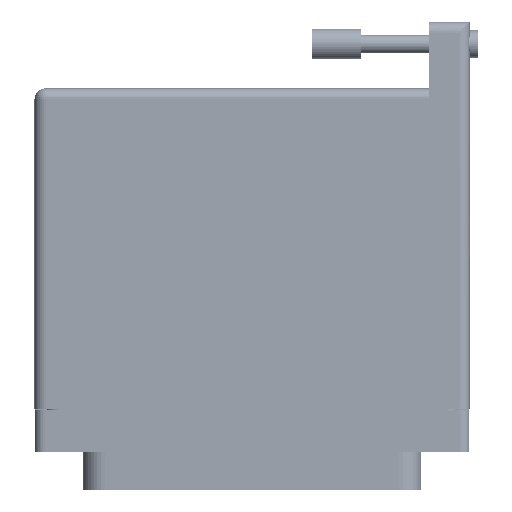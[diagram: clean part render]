
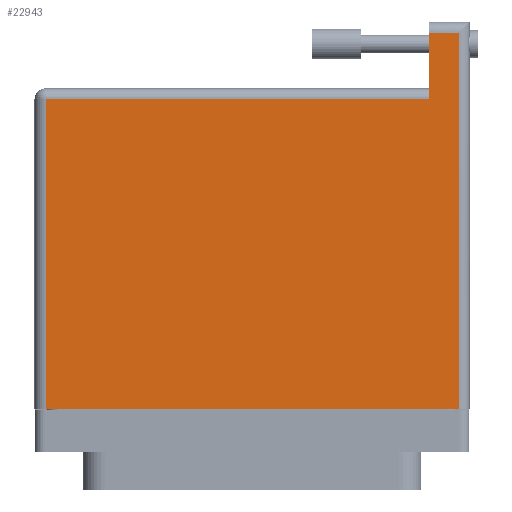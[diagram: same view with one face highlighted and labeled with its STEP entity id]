
A CAD part, front view. The second image highlights one B-rep face of the part: STEP entity #22943.
In plain terms, the highlighted face is planar.
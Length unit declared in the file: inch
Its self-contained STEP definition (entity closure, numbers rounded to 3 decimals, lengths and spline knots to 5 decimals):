
#1358 = DIRECTION ( 'NONE',  ( -1., 0., 0. ) ) ;
#3058 = DIRECTION ( 'NONE',  ( 1., 0., 0. ) ) ;
#5141 = LINE ( 'NONE', #35611, #28770 ) ;
#5504 = CARTESIAN_POINT ( 'NONE',  ( 1.1215, 2.35, 0.765 ) ) ;
#7513 = ORIENTED_EDGE ( 'NONE', *, *, #45523, .T. ) ;
#9622 = VERTEX_POINT ( 'NONE', #56872 ) ;
#10541 = VECTOR ( 'NONE', #24838, 39.37008 ) ;
#12501 = EDGE_LOOP ( 'NONE', ( #52938, #48345, #7513, #20929, #66838, #85293 ) ) ;
#14203 = EDGE_CURVE ( 'NONE', #26260, #32642, #77189, .T. ) ;
#15329 = VERTEX_POINT ( 'NONE', #57240 ) ;
#15358 = VERTEX_POINT ( 'NONE', #23186 ) ;
#20002 = CARTESIAN_POINT ( 'NONE',  ( -1.3075, -0.1, 0.765 ) ) ;
#20929 = ORIENTED_EDGE ( 'NONE', *, *, #73309, .T. ) ;
#22371 = LINE ( 'NONE', #20002, #75187 ) ;
#22452 = CARTESIAN_POINT ( 'NONE',  ( -1.3075, 1.86, 0.765 ) ) ;
#22943 = ADVANCED_FACE ( 'NONE', ( #50663 ), #32079, .F. ) ;
#23186 = CARTESIAN_POINT ( 'NONE',  ( -1.3075, -0.1, 0.765 ) ) ;
#24838 = DIRECTION ( 'NONE',  ( 0., 1., 0. ) ) ;
#25128 = CARTESIAN_POINT ( 'NONE',  ( 1.3075, 2.35, 0.765 ) ) ;
#25647 = CARTESIAN_POINT ( 'NONE',  ( 1.1215, 2.28, 0.765 ) ) ;
#26260 = VERTEX_POINT ( 'NONE', #25647 ) ;
#26635 = DIRECTION ( 'NONE',  ( 0., -1., 0. ) ) ;
#27001 = EDGE_CURVE ( 'NONE', #9622, #26260, #54856, .T. ) ;
#28770 = VECTOR ( 'NONE', #1358, 39.37008 ) ;
#30383 = CARTESIAN_POINT ( 'NONE',  ( -1.3775, -0.1, 0.765 ) ) ;
#32079 = PLANE ( 'NONE',  #88603 ) ;
#32642 = VERTEX_POINT ( 'NONE', #76925 ) ;
#35611 = CARTESIAN_POINT ( 'NONE',  ( -1.3775, 1.86, 0.765 ) ) ;
#39358 = DIRECTION ( 'NONE',  ( -1., 0., 0. ) ) ;
#45307 = EDGE_CURVE ( 'NONE', #15329, #9622, #74166, .T. ) ;
#45523 = EDGE_CURVE ( 'NONE', #67258, #15358, #22371, .T. ) ;
#45669 = EDGE_CURVE ( 'NONE', #32642, #67258, #5141, .T. ) ;
#47859 = DIRECTION ( 'NONE',  ( -1., 0., 0. ) ) ;
#48345 = ORIENTED_EDGE ( 'NONE', *, *, #45669, .T. ) ;
#50663 = FACE_OUTER_BOUND ( 'NONE', #12501, .T. ) ;
#52444 = VECTOR ( 'NONE', #53622, 39.37008 ) ;
#52692 = VECTOR ( 'NONE', #47859, 39.37008 ) ;
#52866 = CARTESIAN_POINT ( 'NONE',  ( -1.3775, 1.93, 0.765 ) ) ;
#52938 = ORIENTED_EDGE ( 'NONE', *, *, #14203, .T. ) ;
#53622 = DIRECTION ( 'NONE',  ( 0., -1., 0. ) ) ;
#54856 = LINE ( 'NONE', #62279, #52692 ) ;
#56872 = CARTESIAN_POINT ( 'NONE',  ( 1.3075, 2.28, 0.765 ) ) ;
#57240 = CARTESIAN_POINT ( 'NONE',  ( 1.3075, -0.1, 0.765 ) ) ;
#62279 = CARTESIAN_POINT ( 'NONE',  ( -1.3775, 2.28, 0.765 ) ) ;
#64922 = LINE ( 'NONE', #30383, #72473 ) ;
#66738 = DIRECTION ( 'NONE',  ( 0., 0., -1. ) ) ;
#66838 = ORIENTED_EDGE ( 'NONE', *, *, #45307, .T. ) ;
#67258 = VERTEX_POINT ( 'NONE', #22452 ) ;
#72473 = VECTOR ( 'NONE', #3058, 39.37008 ) ;
#73309 = EDGE_CURVE ( 'NONE', #15358, #15329, #64922, .T. ) ;
#74166 = LINE ( 'NONE', #25128, #10541 ) ;
#75187 = VECTOR ( 'NONE', #26635, 39.37008 ) ;
#76925 = CARTESIAN_POINT ( 'NONE',  ( 1.1215, 1.86, 0.765 ) ) ;
#77189 = LINE ( 'NONE', #5504, #52444 ) ;
#85293 = ORIENTED_EDGE ( 'NONE', *, *, #27001, .T. ) ;
#88603 = AXIS2_PLACEMENT_3D ( 'NONE', #52866, #66738, #39358 ) ;
